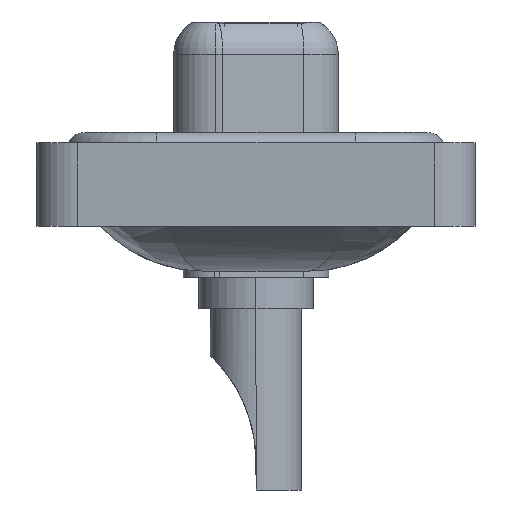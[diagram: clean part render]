
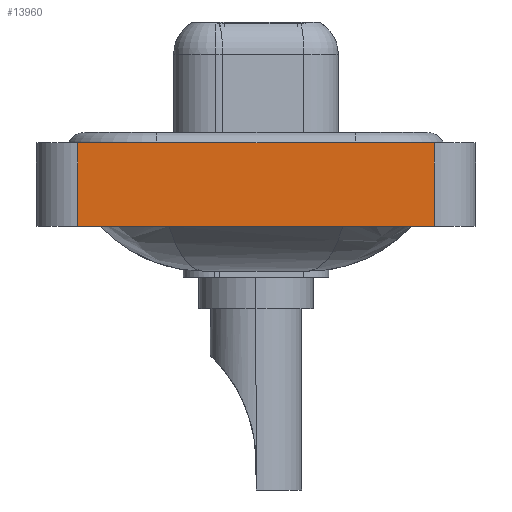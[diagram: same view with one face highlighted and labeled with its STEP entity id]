
A CAD part, left-side view. The second image highlights one B-rep face of the part: STEP entity #13960.
In plain terms, the highlighted planar face has unit normal (-1, 0, 0).
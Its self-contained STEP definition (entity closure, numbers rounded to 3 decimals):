
#246 = VECTOR ( 'NONE', #18957, 1000. ) ;
#272 = DIRECTION ( 'NONE',  ( 0., -1., 0. ) ) ;
#947 = ORIENTED_EDGE ( 'NONE', *, *, #9485, .T. ) ;
#1285 = EDGE_CURVE ( 'NONE', #19975, #10618, #19832, .T. ) ;
#1570 = CARTESIAN_POINT ( 'NONE',  ( -7.35, 8.55, -3.6 ) ) ;
#2037 = PLANE ( 'NONE',  #20163 ) ;
#3597 = CARTESIAN_POINT ( 'NONE',  ( -7.35, -8.55, 0.4 ) ) ;
#3705 = ORIENTED_EDGE ( 'NONE', *, *, #16028, .F. ) ;
#4023 = CARTESIAN_POINT ( 'NONE',  ( -7.35, -8.55, -3.6 ) ) ;
#4261 = CARTESIAN_POINT ( 'NONE',  ( -7.35, -8.55, -3.6 ) ) ;
#6122 = LINE ( 'NONE', #4261, #17586 ) ;
#7349 = ORIENTED_EDGE ( 'NONE', *, *, #1285, .F. ) ;
#7550 = CARTESIAN_POINT ( 'NONE',  ( -7.35, -8.55, 0.4 ) ) ;
#7655 = DIRECTION ( 'NONE',  ( -1., 0., 0. ) ) ;
#7726 = VECTOR ( 'NONE', #8741, 1000. ) ;
#7895 = DIRECTION ( 'NONE',  ( 0., -1., 0. ) ) ;
#8741 = DIRECTION ( 'NONE',  ( 0., 0., 1. ) ) ;
#9485 = EDGE_CURVE ( 'NONE', #19379, #12951, #6122, .T. ) ;
#10618 = VERTEX_POINT ( 'NONE', #3597 ) ;
#10932 = FACE_OUTER_BOUND ( 'NONE', #16214, .T. ) ;
#12951 = VERTEX_POINT ( 'NONE', #21658 ) ;
#13809 = LINE ( 'NONE', #20582, #246 ) ;
#13960 = ADVANCED_FACE ( 'NONE', ( #10932 ), #2037, .T. ) ;
#15658 = LINE ( 'NONE', #1570, #7726 ) ;
#16028 = EDGE_CURVE ( 'NONE', #19379, #19975, #15658, .T. ) ;
#16070 = CARTESIAN_POINT ( 'NONE',  ( -7.35, 8.55, -3.6 ) ) ;
#16194 = VECTOR ( 'NONE', #272, 1000. ) ;
#16214 = EDGE_LOOP ( 'NONE', ( #16960, #7349, #3705, #947 ) ) ;
#16768 = EDGE_CURVE ( 'NONE', #12951, #10618, #13809, .T. ) ;
#16960 = ORIENTED_EDGE ( 'NONE', *, *, #16768, .T. ) ;
#17586 = VECTOR ( 'NONE', #7895, 1000. ) ;
#18957 = DIRECTION ( 'NONE',  ( 0., 0., 1. ) ) ;
#19379 = VERTEX_POINT ( 'NONE', #16070 ) ;
#19832 = LINE ( 'NONE', #7550, #16194 ) ;
#19975 = VERTEX_POINT ( 'NONE', #21754 ) ;
#20163 = AXIS2_PLACEMENT_3D ( 'NONE', #4023, #7655, #21931 ) ;
#20582 = CARTESIAN_POINT ( 'NONE',  ( -7.35, -8.55, -3.6 ) ) ;
#21658 = CARTESIAN_POINT ( 'NONE',  ( -7.35, -8.55, -3.6 ) ) ;
#21754 = CARTESIAN_POINT ( 'NONE',  ( -7.35, 8.55, 0.4 ) ) ;
#21931 = DIRECTION ( 'NONE',  ( 0., 0., 1. ) ) ;
